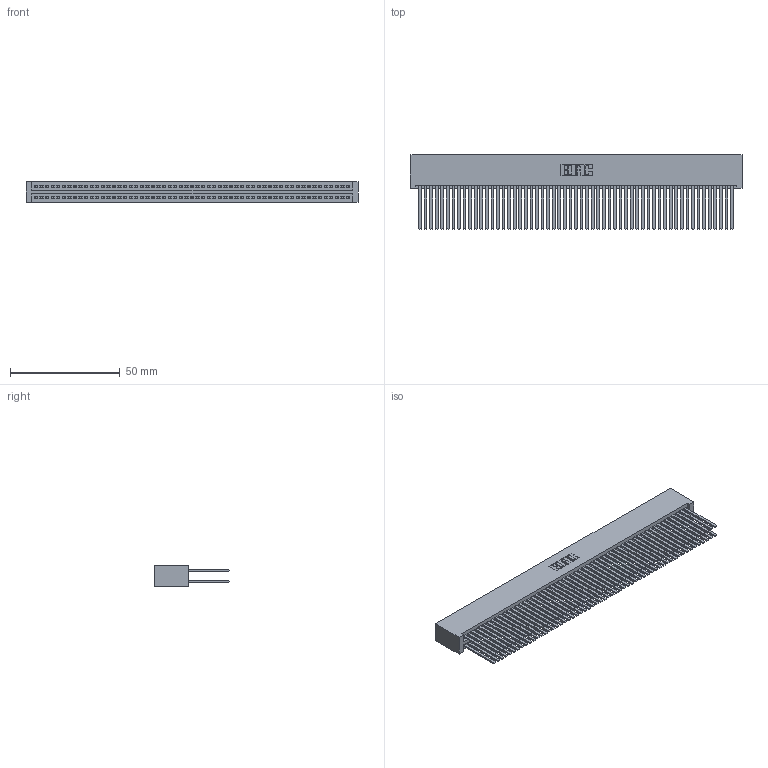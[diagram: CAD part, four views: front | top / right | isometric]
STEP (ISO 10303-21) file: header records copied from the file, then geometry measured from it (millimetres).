
FILE_DESCRIPTION (( 'STEP AP203' ), '1' );
FILE_NAME ('395-114-544-201.STEP', '2019-10-27T18:28:42', ( '' ), ( '' ), 'SwSTEP 2.0', 'SolidWorks 2016', '' );
FILE_SCHEMA (( 'CONFIG_CONTROL_DESIGN' ));
Length unit declared in the file: inch
Products named in the file (3): 345 Part_No Mounting Lugs; 345-292-001_345-293-144; 395-114-544-201
Assembly tree (115 placements, depth 2):
  395-114-544-201
    345 Part_No Mounting Lugs
    345-292-001_345-293-144  x114
Bounding box: 151.38 x 33.96 x 9.4 mm (x, y, z)
Volume: 17058.8 mm3; surface area: 30493.4 mm2
Topology: 115 solids, 115 shells, 5134 faces, 15251 edges, 10014 vertices
Faces by surface type: plane 3382, cylinder 1752
Entity records: 42243 total; most frequent: CARTESIAN_POINT 7064, ORIENTED_EDGE 6998, DIRECTION 6203, EDGE_CURVE 3499, VECTOR 3151, LINE 3151, VERTEX_POINT 2330, AXIS2_PLACEMENT_3D 1526
